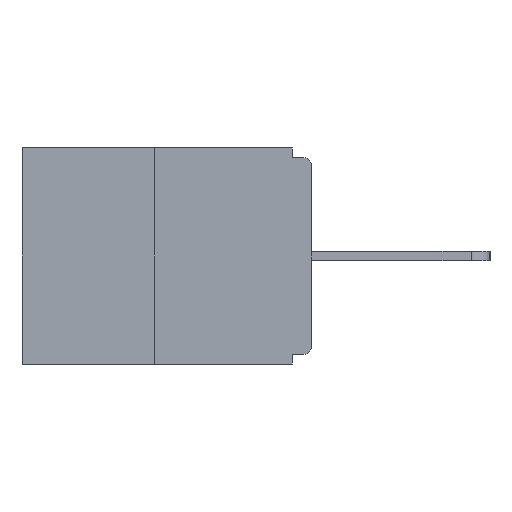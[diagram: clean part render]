
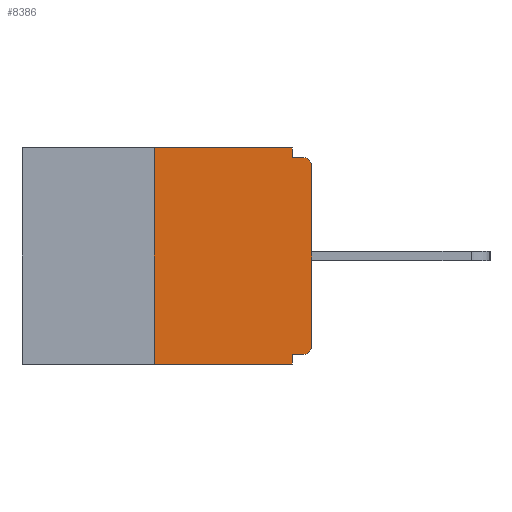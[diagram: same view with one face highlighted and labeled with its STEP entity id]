
A CAD part, left-side view. The second image highlights one B-rep face of the part: STEP entity #8386.
In plain terms, the highlighted planar face has unit normal (-1, 0, 0).
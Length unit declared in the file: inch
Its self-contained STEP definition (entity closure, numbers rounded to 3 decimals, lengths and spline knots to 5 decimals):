
#120 = VERTEX_POINT ( 'NONE', #8171 ) ;
#423 = ORIENTED_EDGE ( 'NONE', *, *, #9129, .F. ) ;
#557 = VECTOR ( 'NONE', #15440, 39.37008 ) ;
#664 = DIRECTION ( 'NONE',  ( 0., -1., 0. ) ) ;
#790 = AXIS2_PLACEMENT_3D ( 'NONE', #10735, #5558, #9549 ) ;
#795 = FACE_OUTER_BOUND ( 'NONE', #9862, .T. ) ;
#1293 = CARTESIAN_POINT ( 'NONE',  ( 0., 0.25, 0. ) ) ;
#1591 = LINE ( 'NONE', #10189, #557 ) ;
#1619 = CARTESIAN_POINT ( 'NONE',  ( 0., 0., -0.328 ) ) ;
#1894 = VECTOR ( 'NONE', #2791, 39.37008 ) ;
#2022 = VERTEX_POINT ( 'NONE', #12338 ) ;
#2382 = ORIENTED_EDGE ( 'NONE', *, *, #8147, .F. ) ;
#2432 = LINE ( 'NONE', #7523, #7468 ) ;
#2455 = AXIS2_PLACEMENT_3D ( 'NONE', #4780, #4872, #7429 ) ;
#2477 = EDGE_CURVE ( 'NONE', #8385, #2022, #15984, .T. ) ;
#2535 = LINE ( 'NONE', #1619, #1894 ) ;
#2545 = VERTEX_POINT ( 'NONE', #1293 ) ;
#2699 = VERTEX_POINT ( 'NONE', #5397 ) ;
#2718 = LINE ( 'NONE', #7798, #13237 ) ;
#2791 = DIRECTION ( 'NONE',  ( 0., 1., 0. ) ) ;
#3425 = CIRCLE ( 'NONE', #790, 0.015 ) ;
#3851 = CARTESIAN_POINT ( 'NONE',  ( 0., 0.031, -0.343 ) ) ;
#3873 = ORIENTED_EDGE ( 'NONE', *, *, #10105, .T. ) ;
#4307 = VECTOR ( 'NONE', #8157, 39.37008 ) ;
#4411 = ORIENTED_EDGE ( 'NONE', *, *, #6586, .T. ) ;
#4649 = CARTESIAN_POINT ( 'NONE',  ( 0., 0., -0.015 ) ) ;
#4730 = EDGE_CURVE ( 'NONE', #6513, #8385, #1591, .T. ) ;
#4780 = CARTESIAN_POINT ( 'NONE',  ( 0., 0.46, 0. ) ) ;
#4849 = ORIENTED_EDGE ( 'NONE', *, *, #6010, .F. ) ;
#4872 = DIRECTION ( 'NONE',  ( 1., 0., 0. ) ) ;
#5124 = VERTEX_POINT ( 'NONE', #15161 ) ;
#5302 = DIRECTION ( 'NONE',  ( 0., 0., 1. ) ) ;
#5397 = CARTESIAN_POINT ( 'NONE',  ( 0., 0., -0.03 ) ) ;
#5437 = EDGE_CURVE ( 'NONE', #120, #8691, #15470, .T. ) ;
#5558 = DIRECTION ( 'NONE',  ( -1., 0., 0. ) ) ;
#6010 = EDGE_CURVE ( 'NONE', #2545, #6513, #2432, .T. ) ;
#6089 = CARTESIAN_POINT ( 'NONE',  ( 0., 0., -0.313 ) ) ;
#6513 = VERTEX_POINT ( 'NONE', #6817 ) ;
#6586 = EDGE_CURVE ( 'NONE', #5124, #14367, #9480, .T. ) ;
#6817 = CARTESIAN_POINT ( 'NONE',  ( 0., 0.031, 0. ) ) ;
#7429 = DIRECTION ( 'NONE',  ( 0., 0., -1. ) ) ;
#7468 = VECTOR ( 'NONE', #12607, 39.37008 ) ;
#7523 = CARTESIAN_POINT ( 'NONE',  ( 0., 0.46, 0. ) ) ;
#7798 = CARTESIAN_POINT ( 'NONE',  ( 0., 0., 0. ) ) ;
#8147 = EDGE_CURVE ( 'NONE', #5124, #2545, #13288, .T. ) ;
#8157 = DIRECTION ( 'NONE',  ( 0., -1., 0. ) ) ;
#8171 = CARTESIAN_POINT ( 'NONE',  ( 0., 0.015, -0.328 ) ) ;
#8266 = ORIENTED_EDGE ( 'NONE', *, *, #4730, .F. ) ;
#8301 = CARTESIAN_POINT ( 'NONE',  ( 0., 0.25, 0. ) ) ;
#8385 = VERTEX_POINT ( 'NONE', #16279 ) ;
#8386 = ADVANCED_FACE ( 'NONE', ( #795 ), #9867, .F. ) ;
#8577 = LINE ( 'NONE', #14672, #10295 ) ;
#8691 = VERTEX_POINT ( 'NONE', #6089 ) ;
#9129 = EDGE_CURVE ( 'NONE', #13091, #14367, #8577, .T. ) ;
#9210 = DIRECTION ( 'NONE',  ( 0., 0., 1. ) ) ;
#9269 = ORIENTED_EDGE ( 'NONE', *, *, #2477, .F. ) ;
#9480 = LINE ( 'NONE', #12073, #13891 ) ;
#9549 = DIRECTION ( 'NONE',  ( 0., 0., -1. ) ) ;
#9604 = AXIS2_PLACEMENT_3D ( 'NONE', #15122, #13777, #16450 ) ;
#9862 = EDGE_LOOP ( 'NONE', ( #4849, #2382, #4411, #423, #10439, #10878, #3873, #11680, #9269, #8266 ) ) ;
#9867 = PLANE ( 'NONE',  #2455 ) ;
#10105 = EDGE_CURVE ( 'NONE', #8691, #2699, #2718, .T. ) ;
#10189 = CARTESIAN_POINT ( 'NONE',  ( 0., 0.031, 0. ) ) ;
#10295 = VECTOR ( 'NONE', #14758, 39.37008 ) ;
#10439 = ORIENTED_EDGE ( 'NONE', *, *, #12810, .F. ) ;
#10723 = VECTOR ( 'NONE', #9210, 39.37008 ) ;
#10735 = CARTESIAN_POINT ( 'NONE',  ( 0., 0.015, -0.03 ) ) ;
#10878 = ORIENTED_EDGE ( 'NONE', *, *, #5437, .T. ) ;
#11316 = EDGE_CURVE ( 'NONE', #2699, #2022, #3425, .T. ) ;
#11680 = ORIENTED_EDGE ( 'NONE', *, *, #11316, .T. ) ;
#12073 = CARTESIAN_POINT ( 'NONE',  ( 0., 0.46, -0.343 ) ) ;
#12338 = CARTESIAN_POINT ( 'NONE',  ( 0., 0.015, -0.015 ) ) ;
#12607 = DIRECTION ( 'NONE',  ( 0., -1., 0. ) ) ;
#12810 = EDGE_CURVE ( 'NONE', #120, #13091, #2535, .T. ) ;
#13091 = VERTEX_POINT ( 'NONE', #13278 ) ;
#13237 = VECTOR ( 'NONE', #5302, 39.37008 ) ;
#13278 = CARTESIAN_POINT ( 'NONE',  ( 0., 0.031, -0.328 ) ) ;
#13288 = LINE ( 'NONE', #8301, #10723 ) ;
#13777 = DIRECTION ( 'NONE',  ( -1., 0., 0. ) ) ;
#13891 = VECTOR ( 'NONE', #664, 39.37008 ) ;
#14367 = VERTEX_POINT ( 'NONE', #3851 ) ;
#14672 = CARTESIAN_POINT ( 'NONE',  ( 0., 0.031, -0.343 ) ) ;
#14758 = DIRECTION ( 'NONE',  ( 0., 0., -1. ) ) ;
#15122 = CARTESIAN_POINT ( 'NONE',  ( 0., 0.015, -0.313 ) ) ;
#15161 = CARTESIAN_POINT ( 'NONE',  ( 0., 0.25, -0.343 ) ) ;
#15440 = DIRECTION ( 'NONE',  ( 0., 0., -1. ) ) ;
#15470 = CIRCLE ( 'NONE', #9604, 0.015 ) ;
#15984 = LINE ( 'NONE', #4649, #4307 ) ;
#16279 = CARTESIAN_POINT ( 'NONE',  ( 0., 0.031, -0.015 ) ) ;
#16450 = DIRECTION ( 'NONE',  ( 0., 0., -1. ) ) ;
